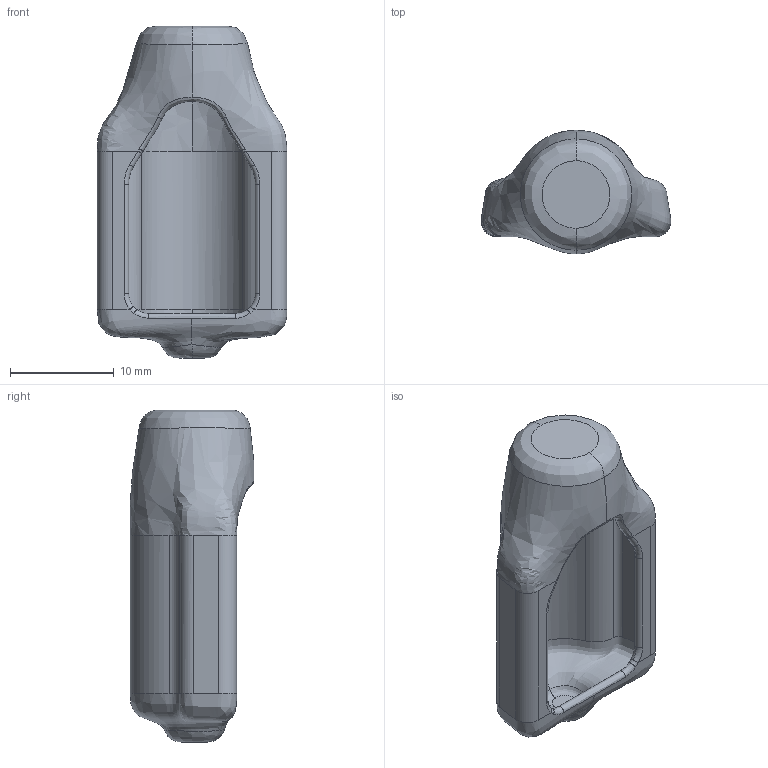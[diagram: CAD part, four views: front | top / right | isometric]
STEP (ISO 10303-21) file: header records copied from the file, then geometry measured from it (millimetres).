
FILE_DESCRIPTION (( 'STEP AP203' ), '1' );
FILE_NAME ('2.2 Hose Clamp Cover NO SUPPORT.STEP', '2022-10-28T16:26:59', ( '' ), ( '' ), 'SwSTEP 2.0', 'SolidWorks 2021', '' );
FILE_SCHEMA (( 'CONFIG_CONTROL_DESIGN' ));
Length unit declared in the file: inch
Products named in the file (1): 2.2 Hose Clamp Cover NO SUPPORT
Bounding box: 18.25 x 11.9 x 31.95 mm (x, y, z)
Volume: 1011.6 mm3; surface area: 2385.4 mm2
Topology: 1 solids, 1 shells, 64 faces, 170 edges, 108 vertices
Faces by surface type: bspline 26, cylinder 18, plane 12, torus 8
Entity records: 45907 total; most frequent: CARTESIAN_POINT 44556, ORIENTED_EDGE 340, EDGE_CURVE 170, DIRECTION 154, VERTEX_POINT 108, B_SPLINE_CURVE_WITH_KNOTS 107, ADVANCED_FACE 64, FACE_OUTER_BOUND 64
